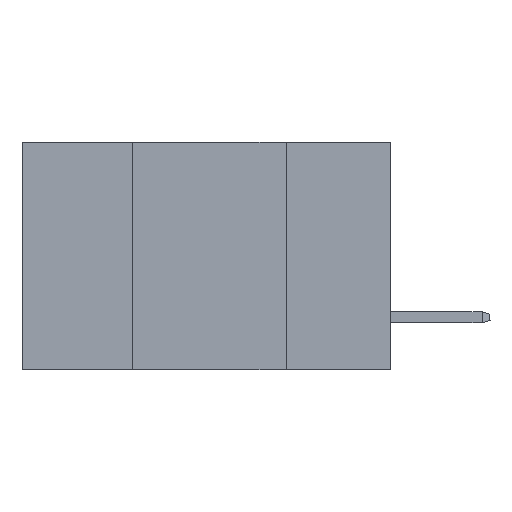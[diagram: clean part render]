
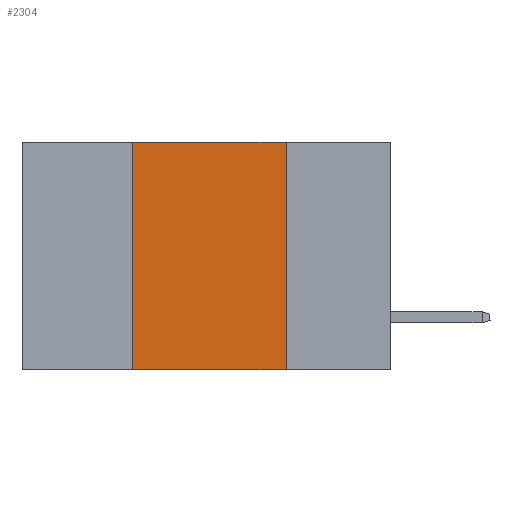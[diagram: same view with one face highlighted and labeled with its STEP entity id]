
A CAD part, left-side view. The second image highlights one B-rep face of the part: STEP entity #2304.
In plain terms, the highlighted planar face has unit normal (-1, 0, 0).
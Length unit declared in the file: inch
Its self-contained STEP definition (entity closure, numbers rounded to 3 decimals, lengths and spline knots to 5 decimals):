
#395 = DIRECTION ( 'NONE',  ( 1., 0., 0. ) ) ;
#477 = FACE_OUTER_BOUND ( 'NONE', #3852, .T. ) ;
#859 = VECTOR ( 'NONE', #6894, 39.37008 ) ;
#997 = DIRECTION ( 'NONE',  ( 0., -1., 0. ) ) ;
#1507 = EDGE_CURVE ( 'NONE', #14982, #2211, #5920, .T. ) ;
#1895 = LINE ( 'NONE', #4658, #14389 ) ;
#2211 = VERTEX_POINT ( 'NONE', #12408 ) ;
#2304 = ADVANCED_FACE ( 'NONE', ( #477 ), #6538, .F. ) ;
#2490 = DIRECTION ( 'NONE',  ( 0., -1., 0. ) ) ;
#2510 = CARTESIAN_POINT ( 'NONE',  ( 0., 0.6, -0.37 ) ) ;
#2859 = VERTEX_POINT ( 'NONE', #6312 ) ;
#3148 = EDGE_CURVE ( 'NONE', #14982, #10491, #10617, .T. ) ;
#3852 = EDGE_LOOP ( 'NONE', ( #10317, #4605, #7844, #5358 ) ) ;
#4326 = AXIS2_PLACEMENT_3D ( 'NONE', #14947, #395, #8985 ) ;
#4605 = ORIENTED_EDGE ( 'NONE', *, *, #10365, .F. ) ;
#4658 = CARTESIAN_POINT ( 'NONE',  ( 0., 0.6, 0. ) ) ;
#5358 = ORIENTED_EDGE ( 'NONE', *, *, #1507, .T. ) ;
#5668 = CARTESIAN_POINT ( 'NONE',  ( 0., 0.42, 0. ) ) ;
#5920 = LINE ( 'NONE', #2510, #14750 ) ;
#6312 = CARTESIAN_POINT ( 'NONE',  ( 0., 0.17, 0. ) ) ;
#6424 = EDGE_CURVE ( 'NONE', #2859, #2211, #15675, .T. ) ;
#6538 = PLANE ( 'NONE',  #4326 ) ;
#6894 = DIRECTION ( 'NONE',  ( 0., 0., 1. ) ) ;
#7844 = ORIENTED_EDGE ( 'NONE', *, *, #3148, .F. ) ;
#8110 = CARTESIAN_POINT ( 'NONE',  ( 0., 0.42, -0.37 ) ) ;
#8985 = DIRECTION ( 'NONE',  ( 0., 0., -1. ) ) ;
#10317 = ORIENTED_EDGE ( 'NONE', *, *, #6424, .F. ) ;
#10365 = EDGE_CURVE ( 'NONE', #10491, #2859, #1895, .T. ) ;
#10491 = VERTEX_POINT ( 'NONE', #10977 ) ;
#10617 = LINE ( 'NONE', #5668, #859 ) ;
#10977 = CARTESIAN_POINT ( 'NONE',  ( 0., 0.42, 0. ) ) ;
#12408 = CARTESIAN_POINT ( 'NONE',  ( 0., 0.17, -0.37 ) ) ;
#13350 = DIRECTION ( 'NONE',  ( 0., 0., -1. ) ) ;
#13454 = CARTESIAN_POINT ( 'NONE',  ( 0., 0.17, 0. ) ) ;
#14389 = VECTOR ( 'NONE', #997, 39.37008 ) ;
#14588 = VECTOR ( 'NONE', #13350, 39.37008 ) ;
#14750 = VECTOR ( 'NONE', #2490, 39.37008 ) ;
#14947 = CARTESIAN_POINT ( 'NONE',  ( 0., 0.6, 0. ) ) ;
#14982 = VERTEX_POINT ( 'NONE', #8110 ) ;
#15675 = LINE ( 'NONE', #13454, #14588 ) ;
